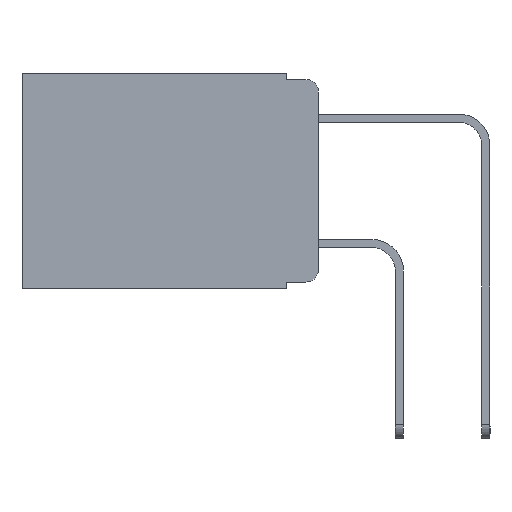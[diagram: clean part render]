
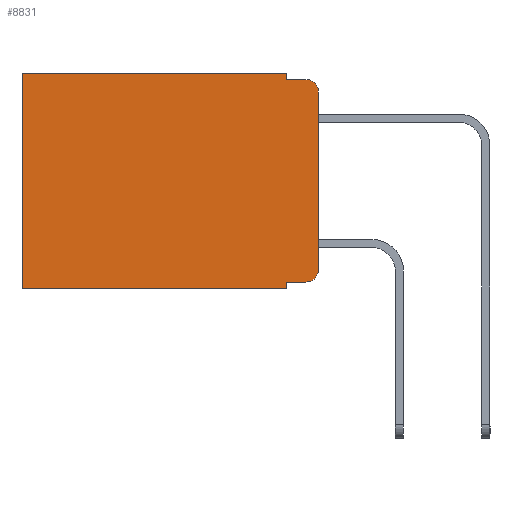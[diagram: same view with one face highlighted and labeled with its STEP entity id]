
A CAD part, left-side view. The second image highlights one B-rep face of the part: STEP entity #8831.
In plain terms, the highlighted planar face has unit normal (-1, 0, 0).
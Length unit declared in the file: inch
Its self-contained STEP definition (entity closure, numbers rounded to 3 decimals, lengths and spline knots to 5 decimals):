
#18 = ORIENTED_EDGE ( 'NONE', *, *, #6874, .T. ) ;
#227 = VERTEX_POINT ( 'NONE', #3284 ) ;
#642 = CARTESIAN_POINT ( 'NONE',  ( 0.298, 0.02, -0.01 ) ) ;
#1137 = LINE ( 'NONE', #14204, #6558 ) ;
#1167 = CARTESIAN_POINT ( 'NONE',  ( 0.298, 0., 0. ) ) ;
#1207 = CARTESIAN_POINT ( 'NONE',  ( 0.298, 0.051, -0.333 ) ) ;
#1221 = VERTEX_POINT ( 'NONE', #1364 ) ;
#1343 = VERTEX_POINT ( 'NONE', #642 ) ;
#1364 = CARTESIAN_POINT ( 'NONE',  ( 0.298, 0., -0.313 ) ) ;
#1372 = LINE ( 'NONE', #1541, #13877 ) ;
#1541 = CARTESIAN_POINT ( 'NONE',  ( 0.298, 0.473, 0. ) ) ;
#1572 = ORIENTED_EDGE ( 'NONE', *, *, #13086, .F. ) ;
#1631 = DIRECTION ( 'NONE',  ( -1., 0., 0. ) ) ;
#2317 = DIRECTION ( 'NONE',  ( 0., 0., -1. ) ) ;
#2425 = CIRCLE ( 'NONE', #15002, 0.02 ) ;
#2619 = DIRECTION ( 'NONE',  ( 0., 0., -1. ) ) ;
#2780 = CARTESIAN_POINT ( 'NONE',  ( 0.298, 0.02, -0.03 ) ) ;
#3039 = AXIS2_PLACEMENT_3D ( 'NONE', #1167, #11861, #9275 ) ;
#3080 = DIRECTION ( 'NONE',  ( 0., 1., 0. ) ) ;
#3235 = CIRCLE ( 'NONE', #6524, 0.02 ) ;
#3284 = CARTESIAN_POINT ( 'NONE',  ( 0.298, 0.473, -0.343 ) ) ;
#3447 = PLANE ( 'NONE',  #3039 ) ;
#3674 = ORIENTED_EDGE ( 'NONE', *, *, #13443, .T. ) ;
#3724 = DIRECTION ( 'NONE',  ( 0., 0., -1. ) ) ;
#3862 = VERTEX_POINT ( 'NONE', #14382 ) ;
#3890 = VERTEX_POINT ( 'NONE', #9713 ) ;
#3942 = LINE ( 'NONE', #11161, #13529 ) ;
#3954 = CARTESIAN_POINT ( 'NONE',  ( 0.298, 0.02, -0.333 ) ) ;
#4147 = LINE ( 'NONE', #13896, #14932 ) ;
#4652 = EDGE_LOOP ( 'NONE', ( #6172, #14702, #1572, #11585, #18, #11893, #13819, #4925, #10530, #3674 ) ) ;
#4925 = ORIENTED_EDGE ( 'NONE', *, *, #7041, .F. ) ;
#5194 = EDGE_CURVE ( 'NONE', #6621, #10426, #5920, .T. ) ;
#5215 = CARTESIAN_POINT ( 'NONE',  ( 0.298, 0.051, -0.01 ) ) ;
#5920 = LINE ( 'NONE', #1207, #8269 ) ;
#6172 = ORIENTED_EDGE ( 'NONE', *, *, #14811, .F. ) ;
#6523 = VECTOR ( 'NONE', #13063, 39.37008 ) ;
#6524 = AXIS2_PLACEMENT_3D ( 'NONE', #2780, #12375, #3724 ) ;
#6558 = VECTOR ( 'NONE', #2317, 39.37008 ) ;
#6621 = VERTEX_POINT ( 'NONE', #15448 ) ;
#6874 = EDGE_CURVE ( 'NONE', #14396, #3890, #10379, .T. ) ;
#7041 = EDGE_CURVE ( 'NONE', #6621, #3862, #8116, .T. ) ;
#7080 = FACE_OUTER_BOUND ( 'NONE', #4652, .T. ) ;
#7800 = DIRECTION ( 'NONE',  ( 0., 0., -1. ) ) ;
#8116 = LINE ( 'NONE', #14257, #6523 ) ;
#8269 = VECTOR ( 'NONE', #15524, 39.37008 ) ;
#8831 = ADVANCED_FACE ( 'NONE', ( #7080 ), #3447, .F. ) ;
#9156 = CARTESIAN_POINT ( 'NONE',  ( 0.298, 0., -0.03 ) ) ;
#9275 = DIRECTION ( 'NONE',  ( 0., 0., -1. ) ) ;
#9646 = EDGE_CURVE ( 'NONE', #3862, #227, #4147, .T. ) ;
#9713 = CARTESIAN_POINT ( 'NONE',  ( 0.298, 0.473, 0. ) ) ;
#10379 = LINE ( 'NONE', #13713, #12025 ) ;
#10426 = VERTEX_POINT ( 'NONE', #3954 ) ;
#10530 = ORIENTED_EDGE ( 'NONE', *, *, #5194, .T. ) ;
#11009 = VERTEX_POINT ( 'NONE', #9156 ) ;
#11161 = CARTESIAN_POINT ( 'NONE',  ( 0.298, 0., 0. ) ) ;
#11175 = DIRECTION ( 'NONE',  ( 0., -1., 0. ) ) ;
#11236 = EDGE_CURVE ( 'NONE', #14396, #15235, #1137, .T. ) ;
#11318 = EDGE_CURVE ( 'NONE', #3890, #227, #1372, .T. ) ;
#11585 = ORIENTED_EDGE ( 'NONE', *, *, #11236, .F. ) ;
#11861 = DIRECTION ( 'NONE',  ( 1., 0., 0. ) ) ;
#11893 = ORIENTED_EDGE ( 'NONE', *, *, #11318, .T. ) ;
#12025 = VECTOR ( 'NONE', #3080, 39.37008 ) ;
#12375 = DIRECTION ( 'NONE',  ( -1., 0., 0. ) ) ;
#12605 = CARTESIAN_POINT ( 'NONE',  ( 0.298, 0.051, 0. ) ) ;
#13063 = DIRECTION ( 'NONE',  ( 0., 0., -1. ) ) ;
#13086 = EDGE_CURVE ( 'NONE', #15235, #1343, #13092, .T. ) ;
#13092 = LINE ( 'NONE', #5215, #13480 ) ;
#13419 = DIRECTION ( 'NONE',  ( 0., 0., -1. ) ) ;
#13443 = EDGE_CURVE ( 'NONE', #10426, #1221, #2425, .T. ) ;
#13480 = VECTOR ( 'NONE', #11175, 39.37008 ) ;
#13529 = VECTOR ( 'NONE', #7800, 39.37008 ) ;
#13675 = CARTESIAN_POINT ( 'NONE',  ( 0.298, 0.02, -0.313 ) ) ;
#13713 = CARTESIAN_POINT ( 'NONE',  ( 0.298, 0., 0. ) ) ;
#13731 = CARTESIAN_POINT ( 'NONE',  ( 0.298, 0.051, -0.01 ) ) ;
#13819 = ORIENTED_EDGE ( 'NONE', *, *, #9646, .F. ) ;
#13877 = VECTOR ( 'NONE', #2619, 39.37008 ) ;
#13896 = CARTESIAN_POINT ( 'NONE',  ( 0.298, 0., -0.343 ) ) ;
#14204 = CARTESIAN_POINT ( 'NONE',  ( 0.298, 0.051, 0. ) ) ;
#14257 = CARTESIAN_POINT ( 'NONE',  ( 0.298, 0.051, 0. ) ) ;
#14382 = CARTESIAN_POINT ( 'NONE',  ( 0.298, 0.051, -0.343 ) ) ;
#14396 = VERTEX_POINT ( 'NONE', #12605 ) ;
#14702 = ORIENTED_EDGE ( 'NONE', *, *, #15478, .T. ) ;
#14811 = EDGE_CURVE ( 'NONE', #11009, #1221, #3942, .T. ) ;
#14932 = VECTOR ( 'NONE', #14995, 39.37008 ) ;
#14995 = DIRECTION ( 'NONE',  ( 0., 1., 0. ) ) ;
#15002 = AXIS2_PLACEMENT_3D ( 'NONE', #13675, #1631, #13419 ) ;
#15235 = VERTEX_POINT ( 'NONE', #13731 ) ;
#15448 = CARTESIAN_POINT ( 'NONE',  ( 0.298, 0.051, -0.333 ) ) ;
#15478 = EDGE_CURVE ( 'NONE', #11009, #1343, #3235, .T. ) ;
#15524 = DIRECTION ( 'NONE',  ( 0., -1., 0. ) ) ;
